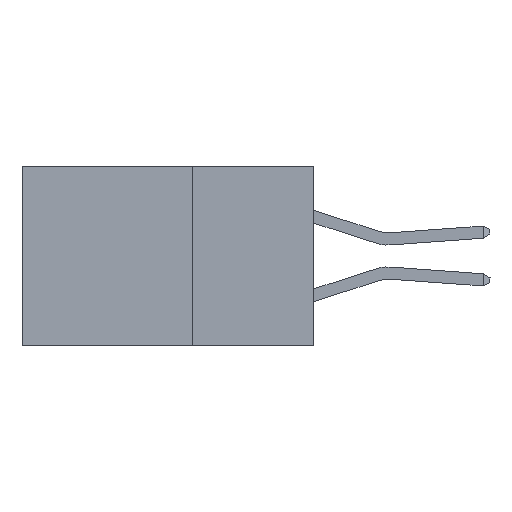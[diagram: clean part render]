
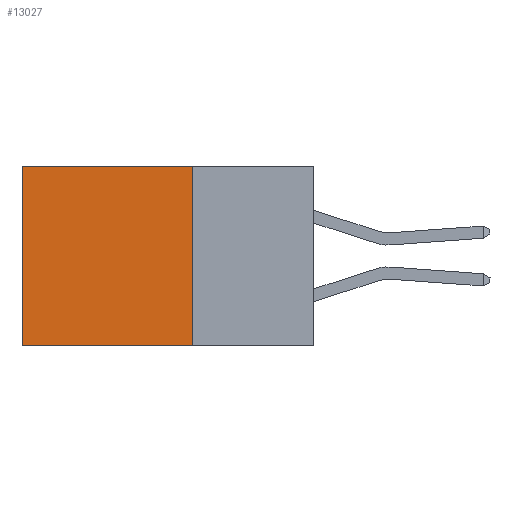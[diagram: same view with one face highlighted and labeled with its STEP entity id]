
A CAD part, left-side view. The second image highlights one B-rep face of the part: STEP entity #13027.
In plain terms, the highlighted planar face has unit normal (-1, 0, 0).
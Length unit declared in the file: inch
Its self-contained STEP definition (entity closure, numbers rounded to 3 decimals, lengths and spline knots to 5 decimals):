
#349 = CARTESIAN_POINT ( 'NONE',  ( 0.2875, 0.25, -0.37 ) ) ;
#1389 = EDGE_CURVE ( 'NONE', #3653, #1825, #16590, .T. ) ;
#1825 = VERTEX_POINT ( 'NONE', #15051 ) ;
#3653 = VERTEX_POINT ( 'NONE', #10878 ) ;
#4056 = VERTEX_POINT ( 'NONE', #18911 ) ;
#4601 = ORIENTED_EDGE ( 'NONE', *, *, #1389, .F. ) ;
#5089 = CARTESIAN_POINT ( 'NONE',  ( 0.2875, 0.25, 0. ) ) ;
#5311 = DIRECTION ( 'NONE',  ( 0., 0., -1. ) ) ;
#5701 = CARTESIAN_POINT ( 'NONE',  ( 0.2875, 0.25, 0. ) ) ;
#5775 = ORIENTED_EDGE ( 'NONE', *, *, #17710, .F. ) ;
#5865 = ORIENTED_EDGE ( 'NONE', *, *, #14755, .T. ) ;
#6182 = VECTOR ( 'NONE', #12820, 39.37008 ) ;
#6243 = EDGE_CURVE ( 'NONE', #10429, #1825, #11174, .T. ) ;
#7956 = VECTOR ( 'NONE', #11365, 39.37008 ) ;
#8359 = PLANE ( 'NONE',  #9802 ) ;
#9802 = AXIS2_PLACEMENT_3D ( 'NONE', #5089, #13823, #5311 ) ;
#10429 = VERTEX_POINT ( 'NONE', #11878 ) ;
#10878 = CARTESIAN_POINT ( 'NONE',  ( 0.2875, 0.25, -0.37 ) ) ;
#11174 = LINE ( 'NONE', #18275, #20659 ) ;
#11365 = DIRECTION ( 'NONE',  ( 0., 1., 0. ) ) ;
#11498 = LINE ( 'NONE', #21925, #17958 ) ;
#11595 = ORIENTED_EDGE ( 'NONE', *, *, #6243, .T. ) ;
#11878 = CARTESIAN_POINT ( 'NONE',  ( 0.2875, 0.6, 0. ) ) ;
#12820 = DIRECTION ( 'NONE',  ( 0., 1., 0. ) ) ;
#13027 = ADVANCED_FACE ( 'NONE', ( #17213 ), #8359, .F. ) ;
#13823 = DIRECTION ( 'NONE',  ( 1., 0., 0. ) ) ;
#14755 = EDGE_CURVE ( 'NONE', #4056, #10429, #21706, .T. ) ;
#15051 = CARTESIAN_POINT ( 'NONE',  ( 0.2875, 0.6, -0.37 ) ) ;
#16590 = LINE ( 'NONE', #349, #7956 ) ;
#16622 = DIRECTION ( 'NONE',  ( 0., 0., -1. ) ) ;
#17213 = FACE_OUTER_BOUND ( 'NONE', #22756, .T. ) ;
#17710 = EDGE_CURVE ( 'NONE', #4056, #3653, #11498, .T. ) ;
#17958 = VECTOR ( 'NONE', #16622, 39.37008 ) ;
#18275 = CARTESIAN_POINT ( 'NONE',  ( 0.2875, 0.6, 0. ) ) ;
#18911 = CARTESIAN_POINT ( 'NONE',  ( 0.2875, 0.25, 0. ) ) ;
#20659 = VECTOR ( 'NONE', #21938, 39.37008 ) ;
#21706 = LINE ( 'NONE', #5701, #6182 ) ;
#21925 = CARTESIAN_POINT ( 'NONE',  ( 0.2875, 0.25, 0. ) ) ;
#21938 = DIRECTION ( 'NONE',  ( 0., 0., -1. ) ) ;
#22756 = EDGE_LOOP ( 'NONE', ( #11595, #4601, #5775, #5865 ) ) ;
